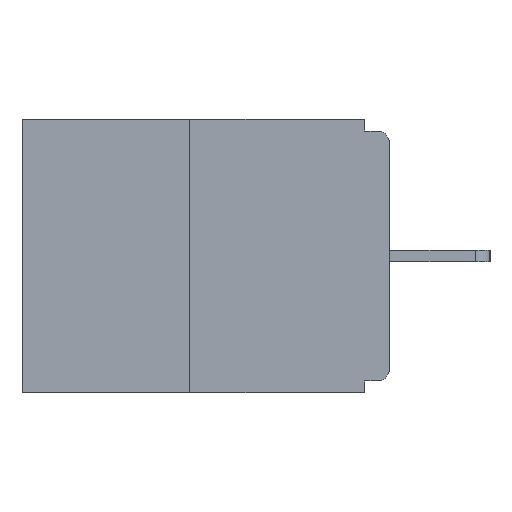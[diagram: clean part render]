
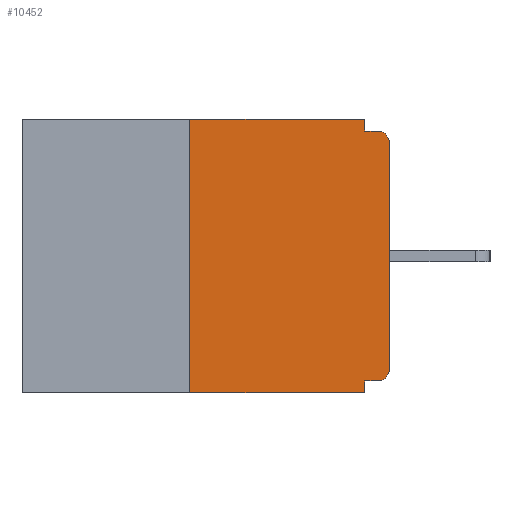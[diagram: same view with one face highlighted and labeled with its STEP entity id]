
A CAD part, left-side view. The second image highlights one B-rep face of the part: STEP entity #10452.
In plain terms, the highlighted planar face has unit normal (-1, 0, 0).
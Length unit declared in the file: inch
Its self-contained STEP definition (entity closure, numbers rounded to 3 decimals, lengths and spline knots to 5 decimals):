
#80 = ORIENTED_EDGE ( 'NONE', *, *, #10366, .T. ) ;
#118 = VERTEX_POINT ( 'NONE', #247 ) ;
#247 = CARTESIAN_POINT ( 'NONE',  ( 0., 0.25, -0.343 ) ) ;
#341 = EDGE_CURVE ( 'NONE', #14465, #8758, #5759, .T. ) ;
#387 = LINE ( 'NONE', #11679, #4985 ) ;
#918 = LINE ( 'NONE', #14762, #11630 ) ;
#990 = CARTESIAN_POINT ( 'NONE',  ( 0., 0.031, 0. ) ) ;
#1111 = VECTOR ( 'NONE', #7950, 39.37008 ) ;
#1421 = CARTESIAN_POINT ( 'NONE',  ( 0., 0.031, -0.343 ) ) ;
#1589 = ORIENTED_EDGE ( 'NONE', *, *, #12474, .F. ) ;
#2138 = EDGE_CURVE ( 'NONE', #15092, #7814, #10378, .T. ) ;
#2532 = CIRCLE ( 'NONE', #5491, 0.015 ) ;
#2646 = ORIENTED_EDGE ( 'NONE', *, *, #14575, .F. ) ;
#3789 = LINE ( 'NONE', #14764, #6398 ) ;
#3870 = VERTEX_POINT ( 'NONE', #15352 ) ;
#3880 = DIRECTION ( 'NONE',  ( 0., -1., 0. ) ) ;
#4253 = ORIENTED_EDGE ( 'NONE', *, *, #2138, .T. ) ;
#4531 = CARTESIAN_POINT ( 'NONE',  ( 0., 0., 0. ) ) ;
#4790 = LINE ( 'NONE', #990, #14064 ) ;
#4938 = CARTESIAN_POINT ( 'NONE',  ( 0., 0.46, 0. ) ) ;
#4985 = VECTOR ( 'NONE', #17036, 39.37008 ) ;
#5112 = LINE ( 'NONE', #4938, #7366 ) ;
#5340 = VERTEX_POINT ( 'NONE', #12043 ) ;
#5343 = VECTOR ( 'NONE', #13305, 39.37008 ) ;
#5371 = CARTESIAN_POINT ( 'NONE',  ( 0., 0.031, -0.328 ) ) ;
#5410 = ORIENTED_EDGE ( 'NONE', *, *, #5638, .T. ) ;
#5491 = AXIS2_PLACEMENT_3D ( 'NONE', #6783, #8342, #12399 ) ;
#5638 = EDGE_CURVE ( 'NONE', #7814, #5340, #17180, .T. ) ;
#5759 = LINE ( 'NONE', #1421, #1111 ) ;
#5793 = VECTOR ( 'NONE', #7040, 39.37008 ) ;
#6398 = VECTOR ( 'NONE', #13579, 39.37008 ) ;
#6783 = CARTESIAN_POINT ( 'NONE',  ( 0., 0.015, -0.03 ) ) ;
#6796 = EDGE_LOOP ( 'NONE', ( #17690, #2646, #14815, #17973, #10439, #4253, #5410, #80, #14383, #1589 ) ) ;
#6945 = VERTEX_POINT ( 'NONE', #10087 ) ;
#7040 = DIRECTION ( 'NONE',  ( 0., 0., 1. ) ) ;
#7270 = CARTESIAN_POINT ( 'NONE',  ( 0., 0.015, -0.313 ) ) ;
#7366 = VECTOR ( 'NONE', #7731, 39.37008 ) ;
#7677 = CARTESIAN_POINT ( 'NONE',  ( 0., 0.031, -0.343 ) ) ;
#7731 = DIRECTION ( 'NONE',  ( 0., -1., 0. ) ) ;
#7814 = VERTEX_POINT ( 'NONE', #16079 ) ;
#7950 = DIRECTION ( 'NONE',  ( 0., 0., -1. ) ) ;
#8228 = CARTESIAN_POINT ( 'NONE',  ( 0., 0.015, -0.328 ) ) ;
#8332 = EDGE_CURVE ( 'NONE', #6945, #10801, #918, .T. ) ;
#8342 = DIRECTION ( 'NONE',  ( -1., 0., 0. ) ) ;
#8530 = DIRECTION ( 'NONE',  ( 0., 0., -1. ) ) ;
#8758 = VERTEX_POINT ( 'NONE', #7677 ) ;
#10087 = CARTESIAN_POINT ( 'NONE',  ( 0., 0.031, -0.015 ) ) ;
#10366 = EDGE_CURVE ( 'NONE', #5340, #10801, #2532, .T. ) ;
#10378 = CIRCLE ( 'NONE', #17439, 0.015 ) ;
#10439 = ORIENTED_EDGE ( 'NONE', *, *, #10692, .F. ) ;
#10452 = ADVANCED_FACE ( 'NONE', ( #16719 ), #12485, .F. ) ;
#10692 = EDGE_CURVE ( 'NONE', #15092, #14465, #3789, .T. ) ;
#10801 = VERTEX_POINT ( 'NONE', #18260 ) ;
#11329 = DIRECTION ( 'NONE',  ( -1., 0., 0. ) ) ;
#11352 = CARTESIAN_POINT ( 'NONE',  ( 0., 0.25, 0. ) ) ;
#11630 = VECTOR ( 'NONE', #3880, 39.37008 ) ;
#11679 = CARTESIAN_POINT ( 'NONE',  ( 0., 0.46, -0.343 ) ) ;
#12043 = CARTESIAN_POINT ( 'NONE',  ( 0., 0., -0.03 ) ) ;
#12399 = DIRECTION ( 'NONE',  ( 0., 0., -1. ) ) ;
#12474 = EDGE_CURVE ( 'NONE', #3870, #6945, #4790, .T. ) ;
#12485 = PLANE ( 'NONE',  #13764 ) ;
#12518 = DIRECTION ( 'NONE',  ( 0., 0., -1. ) ) ;
#13305 = DIRECTION ( 'NONE',  ( 0., 0., 1. ) ) ;
#13579 = DIRECTION ( 'NONE',  ( 0., 1., 0. ) ) ;
#13764 = AXIS2_PLACEMENT_3D ( 'NONE', #16900, #14139, #8530 ) ;
#13945 = LINE ( 'NONE', #16706, #5793 ) ;
#14064 = VECTOR ( 'NONE', #16405, 39.37008 ) ;
#14139 = DIRECTION ( 'NONE',  ( 1., 0., 0. ) ) ;
#14383 = ORIENTED_EDGE ( 'NONE', *, *, #8332, .F. ) ;
#14465 = VERTEX_POINT ( 'NONE', #5371 ) ;
#14575 = EDGE_CURVE ( 'NONE', #118, #15065, #13945, .T. ) ;
#14762 = CARTESIAN_POINT ( 'NONE',  ( 0., 0., -0.015 ) ) ;
#14764 = CARTESIAN_POINT ( 'NONE',  ( 0., 0., -0.328 ) ) ;
#14815 = ORIENTED_EDGE ( 'NONE', *, *, #18128, .T. ) ;
#15065 = VERTEX_POINT ( 'NONE', #11352 ) ;
#15092 = VERTEX_POINT ( 'NONE', #8228 ) ;
#15352 = CARTESIAN_POINT ( 'NONE',  ( 0., 0.031, 0. ) ) ;
#16079 = CARTESIAN_POINT ( 'NONE',  ( 0., 0., -0.313 ) ) ;
#16405 = DIRECTION ( 'NONE',  ( 0., 0., -1. ) ) ;
#16706 = CARTESIAN_POINT ( 'NONE',  ( 0., 0.25, 0. ) ) ;
#16719 = FACE_OUTER_BOUND ( 'NONE', #6796, .T. ) ;
#16900 = CARTESIAN_POINT ( 'NONE',  ( 0., 0.46, 0. ) ) ;
#17036 = DIRECTION ( 'NONE',  ( 0., -1., 0. ) ) ;
#17180 = LINE ( 'NONE', #4531, #5343 ) ;
#17439 = AXIS2_PLACEMENT_3D ( 'NONE', #7270, #11329, #12518 ) ;
#17690 = ORIENTED_EDGE ( 'NONE', *, *, #18256, .F. ) ;
#17973 = ORIENTED_EDGE ( 'NONE', *, *, #341, .F. ) ;
#18128 = EDGE_CURVE ( 'NONE', #118, #8758, #387, .T. ) ;
#18256 = EDGE_CURVE ( 'NONE', #15065, #3870, #5112, .T. ) ;
#18260 = CARTESIAN_POINT ( 'NONE',  ( 0., 0.015, -0.015 ) ) ;
